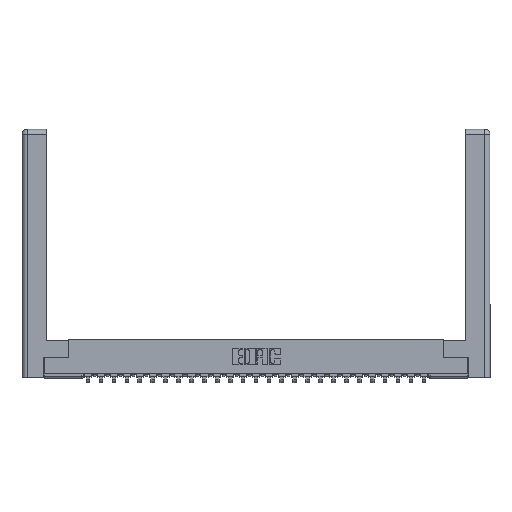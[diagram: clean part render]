
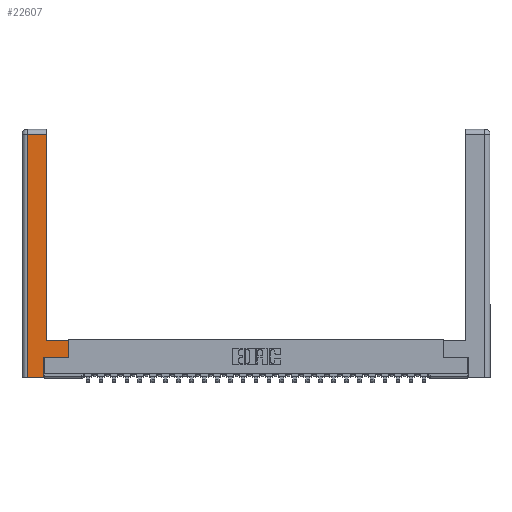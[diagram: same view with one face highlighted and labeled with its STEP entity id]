
A CAD part, top view. The second image highlights one B-rep face of the part: STEP entity #22607.
In plain terms, the highlighted planar face has unit normal (0, 0, 1).
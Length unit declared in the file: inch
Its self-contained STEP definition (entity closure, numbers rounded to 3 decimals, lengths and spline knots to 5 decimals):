
#93 = CARTESIAN_POINT ( 'NONE',  ( 0.0615, 0., 0. ) ) ;
#335 = VECTOR ( 'NONE', #25086, 39.37008 ) ;
#568 = DIRECTION ( 'NONE',  ( -1., 0., 0. ) ) ;
#831 = CARTESIAN_POINT ( 'NONE',  ( 0.265, 0., 0. ) ) ;
#1548 = CARTESIAN_POINT ( 'NONE',  ( 0.295, 0.45, 0. ) ) ;
#1708 = VERTEX_POINT ( 'NONE', #1548 ) ;
#1935 = VECTOR ( 'NONE', #17848, 39.37008 ) ;
#2274 = LINE ( 'NONE', #2410, #22052 ) ;
#2327 = FACE_OUTER_BOUND ( 'NONE', #25212, .T. ) ;
#2410 = CARTESIAN_POINT ( 'NONE',  ( 0.295, 0.45, 0. ) ) ;
#3088 = CARTESIAN_POINT ( 'NONE',  ( 0.565, 0.45, 0. ) ) ;
#3093 = LINE ( 'NONE', #20544, #18877 ) ;
#3486 = VERTEX_POINT ( 'NONE', #3088 ) ;
#3522 = EDGE_CURVE ( 'NONE', #17154, #7748, #5238, .T. ) ;
#3995 = LINE ( 'NONE', #93, #1935 ) ;
#4040 = VECTOR ( 'NONE', #12077, 39.37008 ) ;
#4411 = EDGE_CURVE ( 'NONE', #21597, #17154, #3093, .T. ) ;
#4902 = LINE ( 'NONE', #13693, #26198 ) ;
#5238 = LINE ( 'NONE', #18535, #14850 ) ;
#5347 = EDGE_CURVE ( 'NONE', #8064, #26366, #4902, .T. ) ;
#6316 = AXIS2_PLACEMENT_3D ( 'NONE', #17763, #13274, #6928 ) ;
#6928 = DIRECTION ( 'NONE',  ( -1., 0., 0. ) ) ;
#7058 = ORIENTED_EDGE ( 'NONE', *, *, #3522, .T. ) ;
#7194 = CARTESIAN_POINT ( 'NONE',  ( 0.0615, 2.94, 0. ) ) ;
#7748 = VERTEX_POINT ( 'NONE', #17516 ) ;
#8064 = VERTEX_POINT ( 'NONE', #9574 ) ;
#8134 = LINE ( 'NONE', #28012, #27062 ) ;
#9574 = CARTESIAN_POINT ( 'NONE',  ( 0.295, 2.94, 0. ) ) ;
#11792 = LINE ( 'NONE', #831, #4040 ) ;
#11879 = DIRECTION ( 'NONE',  ( 1., 0., 0. ) ) ;
#12077 = DIRECTION ( 'NONE',  ( 1., 0., 0. ) ) ;
#12345 = ORIENTED_EDGE ( 'NONE', *, *, #25379, .T. ) ;
#12525 = CARTESIAN_POINT ( 'NONE',  ( 0.295, 3., 0. ) ) ;
#13274 = DIRECTION ( 'NONE',  ( 0., 0., -1. ) ) ;
#13693 = CARTESIAN_POINT ( 'NONE',  ( 0.0615, 2.94, 0. ) ) ;
#13700 = PLANE ( 'NONE',  #6316 ) ;
#14649 = EDGE_CURVE ( 'NONE', #26366, #20168, #3995, .T. ) ;
#14850 = VECTOR ( 'NONE', #11879, 39.37008 ) ;
#15371 = CARTESIAN_POINT ( 'NONE',  ( 0.265, 0., 0. ) ) ;
#16292 = ORIENTED_EDGE ( 'NONE', *, *, #24452, .T. ) ;
#17154 = VERTEX_POINT ( 'NONE', #22996 ) ;
#17516 = CARTESIAN_POINT ( 'NONE',  ( 0.565, 0.245, 0. ) ) ;
#17763 = CARTESIAN_POINT ( 'NONE',  ( 0., 0., 0. ) ) ;
#17779 = ORIENTED_EDGE ( 'NONE', *, *, #14649, .T. ) ;
#17848 = DIRECTION ( 'NONE',  ( 0., -1., 0. ) ) ;
#18535 = CARTESIAN_POINT ( 'NONE',  ( 0.565, 0.245, 0. ) ) ;
#18877 = VECTOR ( 'NONE', #20694, 39.37008 ) ;
#20168 = VERTEX_POINT ( 'NONE', #21133 ) ;
#20453 = ORIENTED_EDGE ( 'NONE', *, *, #24031, .T. ) ;
#20544 = CARTESIAN_POINT ( 'NONE',  ( 0.265, 0.245, 0. ) ) ;
#20694 = DIRECTION ( 'NONE',  ( 0., 1., 0. ) ) ;
#21133 = CARTESIAN_POINT ( 'NONE',  ( 0.0615, 0., 0. ) ) ;
#21561 = DIRECTION ( 'NONE',  ( 0., 1., 0. ) ) ;
#21597 = VERTEX_POINT ( 'NONE', #15371 ) ;
#22052 = VECTOR ( 'NONE', #28353, 39.37008 ) ;
#22607 = ADVANCED_FACE ( 'NONE', ( #2327 ), #13700, .F. ) ;
#22996 = CARTESIAN_POINT ( 'NONE',  ( 0.265, 0.245, 0. ) ) ;
#23265 = EDGE_CURVE ( 'NONE', #7748, #3486, #8134, .T. ) ;
#23506 = LINE ( 'NONE', #12525, #335 ) ;
#24031 = EDGE_CURVE ( 'NONE', #1708, #8064, #23506, .T. ) ;
#24197 = ORIENTED_EDGE ( 'NONE', *, *, #23265, .T. ) ;
#24452 = EDGE_CURVE ( 'NONE', #20168, #21597, #11792, .T. ) ;
#25086 = DIRECTION ( 'NONE',  ( 0., 1., 0. ) ) ;
#25212 = EDGE_LOOP ( 'NONE', ( #20453, #26763, #17779, #16292, #25706, #7058, #24197, #12345 ) ) ;
#25379 = EDGE_CURVE ( 'NONE', #3486, #1708, #2274, .T. ) ;
#25706 = ORIENTED_EDGE ( 'NONE', *, *, #4411, .T. ) ;
#26198 = VECTOR ( 'NONE', #568, 39.37008 ) ;
#26366 = VERTEX_POINT ( 'NONE', #7194 ) ;
#26763 = ORIENTED_EDGE ( 'NONE', *, *, #5347, .T. ) ;
#27062 = VECTOR ( 'NONE', #21561, 39.37008 ) ;
#28012 = CARTESIAN_POINT ( 'NONE',  ( 0.565, 0.45, 0. ) ) ;
#28353 = DIRECTION ( 'NONE',  ( -1., 0., 0. ) ) ;
